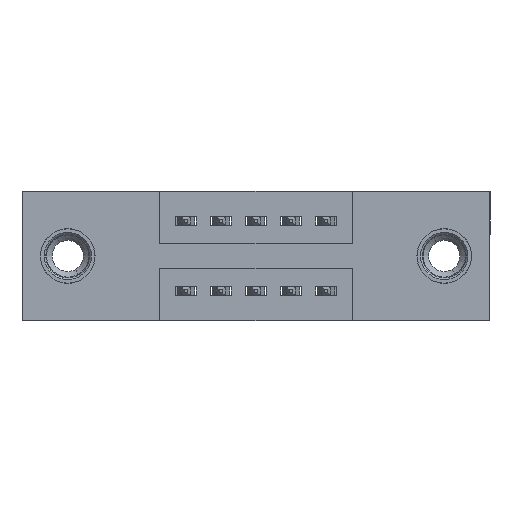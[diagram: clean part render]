
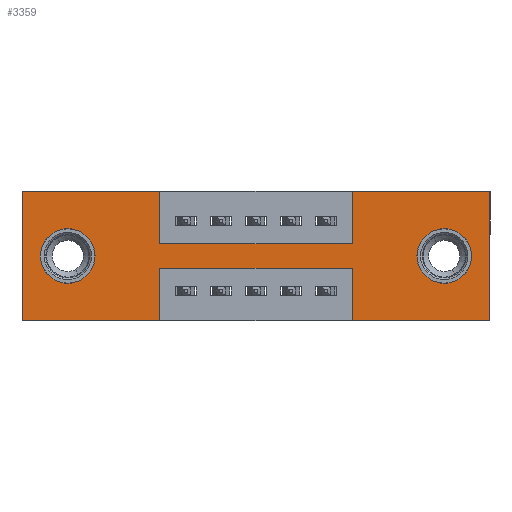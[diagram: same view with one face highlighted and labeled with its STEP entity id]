
A CAD part, front view. The second image highlights one B-rep face of the part: STEP entity #3359.
In plain terms, the highlighted planar face has unit normal (0, -1, 0).
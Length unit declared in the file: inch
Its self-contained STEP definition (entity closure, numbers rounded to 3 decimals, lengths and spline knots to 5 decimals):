
#49 = CIRCLE ( 'NONE', #4839, 0.078 ) ;
#59 = CIRCLE ( 'NONE', #9215, 0.078 ) ;
#91 = VECTOR ( 'NONE', #526, 39.37008 ) ;
#141 = EDGE_CURVE ( 'NONE', #2219, #10089, #9930, .T. ) ;
#295 = CARTESIAN_POINT ( 'NONE',  ( 0.9425, 0., 0. ) ) ;
#468 = EDGE_CURVE ( 'NONE', #2210, #6385, #59, .T. ) ;
#486 = CARTESIAN_POINT ( 'NONE',  ( 0.3925, 0., -0.15 ) ) ;
#526 = DIRECTION ( 'NONE',  ( 1., 0., 0. ) ) ;
#622 = VERTEX_POINT ( 'NONE', #5616 ) ;
#686 = CARTESIAN_POINT ( 'NONE',  ( 0.3925, 0., -0.22 ) ) ;
#697 = CARTESIAN_POINT ( 'NONE',  ( 0.9425, 0., -0.37 ) ) ;
#868 = DIRECTION ( 'NONE',  ( 1., 0., 0. ) ) ;
#916 = DIRECTION ( 'NONE',  ( 0., 1., 0. ) ) ;
#958 = AXIS2_PLACEMENT_3D ( 'NONE', #9593, #4561, #10365 ) ;
#1003 = EDGE_CURVE ( 'NONE', #6385, #2210, #49, .T. ) ;
#1082 = ORIENTED_EDGE ( 'NONE', *, *, #10305, .F. ) ;
#1148 = EDGE_CURVE ( 'NONE', #7200, #5739, #3482, .T. ) ;
#1310 = CARTESIAN_POINT ( 'NONE',  ( 0.9425, 0., 0. ) ) ;
#1351 = DIRECTION ( 'NONE',  ( 0., 0., -1. ) ) ;
#1407 = LINE ( 'NONE', #5954, #10158 ) ;
#1482 = CARTESIAN_POINT ( 'NONE',  ( 0., 0., 0. ) ) ;
#1580 = DIRECTION ( 'NONE',  ( 0., 0., -1. ) ) ;
#1800 = CARTESIAN_POINT ( 'NONE',  ( 0.3925, 0., -0.15 ) ) ;
#1824 = CARTESIAN_POINT ( 'NONE',  ( 0.13, 0., -0.107 ) ) ;
#1929 = EDGE_CURVE ( 'NONE', #622, #3042, #7512, .T. ) ;
#1952 = CARTESIAN_POINT ( 'NONE',  ( 0.9425, 0., -0.37 ) ) ;
#1994 = CIRCLE ( 'NONE', #958, 0.078 ) ;
#2064 = DIRECTION ( 'NONE',  ( 0., 1., 0. ) ) ;
#2210 = VERTEX_POINT ( 'NONE', #9227 ) ;
#2219 = VERTEX_POINT ( 'NONE', #4919 ) ;
#2339 = ORIENTED_EDGE ( 'NONE', *, *, #7412, .F. ) ;
#2413 = FACE_OUTER_BOUND ( 'NONE', #6311, .T. ) ;
#2610 = EDGE_CURVE ( 'NONE', #4002, #9605, #7363, .T. ) ;
#2875 = EDGE_CURVE ( 'NONE', #3719, #6093, #9187, .T. ) ;
#3030 = EDGE_CURVE ( 'NONE', #5972, #3719, #5895, .T. ) ;
#3042 = VERTEX_POINT ( 'NONE', #1800 ) ;
#3090 = VECTOR ( 'NONE', #9256, 39.37008 ) ;
#3156 = DIRECTION ( 'NONE',  ( 0., 0., 1. ) ) ;
#3162 = EDGE_CURVE ( 'NONE', #6093, #5777, #6832, .T. ) ;
#3178 = EDGE_CURVE ( 'NONE', #5739, #7200, #1994, .T. ) ;
#3226 = VECTOR ( 'NONE', #6180, 39.37008 ) ;
#3320 = ORIENTED_EDGE ( 'NONE', *, *, #2875, .F. ) ;
#3359 = ADVANCED_FACE ( 'NONE', ( #4691, #11044, #2413 ), #3971, .T. ) ;
#3482 = CIRCLE ( 'NONE', #9891, 0.078 ) ;
#3538 = VECTOR ( 'NONE', #4906, 39.37008 ) ;
#3704 = ORIENTED_EDGE ( 'NONE', *, *, #3162, .F. ) ;
#3719 = VERTEX_POINT ( 'NONE', #8598 ) ;
#3761 = ORIENTED_EDGE ( 'NONE', *, *, #8910, .F. ) ;
#3765 = VERTEX_POINT ( 'NONE', #7660 ) ;
#3971 = PLANE ( 'NONE',  #9531 ) ;
#3981 = LINE ( 'NONE', #295, #7941 ) ;
#4002 = VERTEX_POINT ( 'NONE', #4796 ) ;
#4092 = DIRECTION ( 'NONE',  ( 0., 0., -1. ) ) ;
#4152 = EDGE_CURVE ( 'NONE', #10089, #3765, #10294, .T. ) ;
#4168 = EDGE_CURVE ( 'NONE', #9605, #622, #5368, .T. ) ;
#4209 = CARTESIAN_POINT ( 'NONE',  ( 0., 0., 0. ) ) ;
#4366 = DIRECTION ( 'NONE',  ( 0., 0., 1. ) ) ;
#4561 = DIRECTION ( 'NONE',  ( 0., 1., 0. ) ) ;
#4691 = FACE_BOUND ( 'NONE', #7222, .T. ) ;
#4723 = DIRECTION ( 'NONE',  ( 0., 0., 1. ) ) ;
#4785 = ORIENTED_EDGE ( 'NONE', *, *, #6636, .F. ) ;
#4796 = CARTESIAN_POINT ( 'NONE',  ( 0., 0., -0.37 ) ) ;
#4839 = AXIS2_PLACEMENT_3D ( 'NONE', #8988, #6230, #4366 ) ;
#4844 = LINE ( 'NONE', #486, #91 ) ;
#4906 = DIRECTION ( 'NONE',  ( 0., 0., -1. ) ) ;
#4919 = CARTESIAN_POINT ( 'NONE',  ( 0.9425, 0., -0.22 ) ) ;
#5107 = VECTOR ( 'NONE', #7094, 39.37008 ) ;
#5187 = CARTESIAN_POINT ( 'NONE',  ( 0.3925, 0., 0. ) ) ;
#5346 = CARTESIAN_POINT ( 'NONE',  ( 1.205, 0., -0.263 ) ) ;
#5353 = ORIENTED_EDGE ( 'NONE', *, *, #468, .T. ) ;
#5368 = LINE ( 'NONE', #4209, #3090 ) ;
#5616 = CARTESIAN_POINT ( 'NONE',  ( 0.3925, 0., 0. ) ) ;
#5625 = VECTOR ( 'NONE', #1580, 39.37008 ) ;
#5739 = VERTEX_POINT ( 'NONE', #5346 ) ;
#5777 = VERTEX_POINT ( 'NONE', #1952 ) ;
#5895 = LINE ( 'NONE', #9422, #9816 ) ;
#5926 = EDGE_LOOP ( 'NONE', ( #6222, #5353 ) ) ;
#5954 = CARTESIAN_POINT ( 'NONE',  ( 0., 0., -0.37 ) ) ;
#5972 = VERTEX_POINT ( 'NONE', #1310 ) ;
#6093 = VERTEX_POINT ( 'NONE', #7480 ) ;
#6180 = DIRECTION ( 'NONE',  ( -1., 0., 0. ) ) ;
#6222 = ORIENTED_EDGE ( 'NONE', *, *, #1003, .T. ) ;
#6230 = DIRECTION ( 'NONE',  ( 0., 1., 0. ) ) ;
#6311 = EDGE_LOOP ( 'NONE', ( #6622, #6371, #2339, #3704, #3320, #9814, #4785, #3761, #8026, #6798, #6451, #1082 ) ) ;
#6346 = CARTESIAN_POINT ( 'NONE',  ( 1.205, 0., -0.185 ) ) ;
#6371 = ORIENTED_EDGE ( 'NONE', *, *, #141, .F. ) ;
#6385 = VERTEX_POINT ( 'NONE', #1824 ) ;
#6451 = ORIENTED_EDGE ( 'NONE', *, *, #2610, .F. ) ;
#6539 = DIRECTION ( 'NONE',  ( 0., -1., 0. ) ) ;
#6575 = VECTOR ( 'NONE', #10340, 39.37008 ) ;
#6622 = ORIENTED_EDGE ( 'NONE', *, *, #4152, .F. ) ;
#6636 = EDGE_CURVE ( 'NONE', #8568, #5972, #3981, .T. ) ;
#6744 = CARTESIAN_POINT ( 'NONE',  ( 0.3925, 0., -0.37 ) ) ;
#6765 = DIRECTION ( 'NONE',  ( 0., 0., 1. ) ) ;
#6798 = ORIENTED_EDGE ( 'NONE', *, *, #4168, .F. ) ;
#6817 = DIRECTION ( 'NONE',  ( -1., 0., 0. ) ) ;
#6832 = LINE ( 'NONE', #8710, #6575 ) ;
#6975 = VECTOR ( 'NONE', #8250, 39.37008 ) ;
#7017 = VECTOR ( 'NONE', #6765, 39.37008 ) ;
#7094 = DIRECTION ( 'NONE',  ( 0., 0., 1. ) ) ;
#7200 = VERTEX_POINT ( 'NONE', #7237 ) ;
#7222 = EDGE_LOOP ( 'NONE', ( #9535, #9199 ) ) ;
#7237 = CARTESIAN_POINT ( 'NONE',  ( 1.205, 0., -0.107 ) ) ;
#7363 = LINE ( 'NONE', #10345, #5107 ) ;
#7412 = EDGE_CURVE ( 'NONE', #5777, #2219, #9491, .T. ) ;
#7416 = CARTESIAN_POINT ( 'NONE',  ( 1.335, 0., 0. ) ) ;
#7480 = CARTESIAN_POINT ( 'NONE',  ( 1.335, 0., -0.37 ) ) ;
#7512 = LINE ( 'NONE', #5187, #3538 ) ;
#7660 = CARTESIAN_POINT ( 'NONE',  ( 0.3925, 0., -0.37 ) ) ;
#7847 = CARTESIAN_POINT ( 'NONE',  ( 0.9425, 0., -0.15 ) ) ;
#7941 = VECTOR ( 'NONE', #4723, 39.37008 ) ;
#8026 = ORIENTED_EDGE ( 'NONE', *, *, #1929, .F. ) ;
#8250 = DIRECTION ( 'NONE',  ( 0., 0., -1. ) ) ;
#8568 = VERTEX_POINT ( 'NONE', #7847 ) ;
#8598 = CARTESIAN_POINT ( 'NONE',  ( 1.335, 0., 0. ) ) ;
#8710 = CARTESIAN_POINT ( 'NONE',  ( 0., 0., -0.37 ) ) ;
#8910 = EDGE_CURVE ( 'NONE', #3042, #8568, #4844, .T. ) ;
#8988 = CARTESIAN_POINT ( 'NONE',  ( 0.13, 0., -0.185 ) ) ;
#9002 = CARTESIAN_POINT ( 'NONE',  ( 0.3925, 0., -0.22 ) ) ;
#9187 = LINE ( 'NONE', #7416, #6975 ) ;
#9199 = ORIENTED_EDGE ( 'NONE', *, *, #3178, .T. ) ;
#9215 = AXIS2_PLACEMENT_3D ( 'NONE', #9345, #916, #3156 ) ;
#9227 = CARTESIAN_POINT ( 'NONE',  ( 0.13, 0., -0.263 ) ) ;
#9256 = DIRECTION ( 'NONE',  ( 1., 0., 0. ) ) ;
#9345 = CARTESIAN_POINT ( 'NONE',  ( 0.13, 0., -0.185 ) ) ;
#9422 = CARTESIAN_POINT ( 'NONE',  ( 0., 0., 0. ) ) ;
#9491 = LINE ( 'NONE', #697, #7017 ) ;
#9531 = AXIS2_PLACEMENT_3D ( 'NONE', #10621, #6539, #1351 ) ;
#9535 = ORIENTED_EDGE ( 'NONE', *, *, #1148, .T. ) ;
#9593 = CARTESIAN_POINT ( 'NONE',  ( 1.205, 0., -0.185 ) ) ;
#9605 = VERTEX_POINT ( 'NONE', #1482 ) ;
#9814 = ORIENTED_EDGE ( 'NONE', *, *, #3030, .F. ) ;
#9816 = VECTOR ( 'NONE', #868, 39.37008 ) ;
#9891 = AXIS2_PLACEMENT_3D ( 'NONE', #6346, #2064, #4092 ) ;
#9930 = LINE ( 'NONE', #686, #3226 ) ;
#10089 = VERTEX_POINT ( 'NONE', #9002 ) ;
#10158 = VECTOR ( 'NONE', #6817, 39.37008 ) ;
#10294 = LINE ( 'NONE', #6744, #5625 ) ;
#10305 = EDGE_CURVE ( 'NONE', #3765, #4002, #1407, .T. ) ;
#10340 = DIRECTION ( 'NONE',  ( -1., 0., 0. ) ) ;
#10345 = CARTESIAN_POINT ( 'NONE',  ( 0., 0., 0. ) ) ;
#10365 = DIRECTION ( 'NONE',  ( 0., 0., -1. ) ) ;
#10621 = CARTESIAN_POINT ( 'NONE',  ( 0., 0., -0.37 ) ) ;
#11044 = FACE_BOUND ( 'NONE', #5926, .T. ) ;
